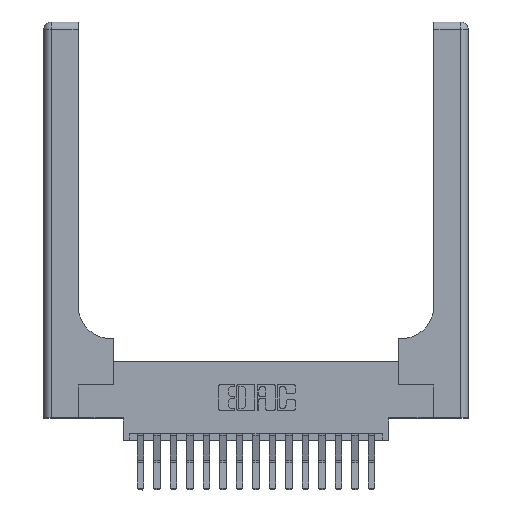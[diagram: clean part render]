
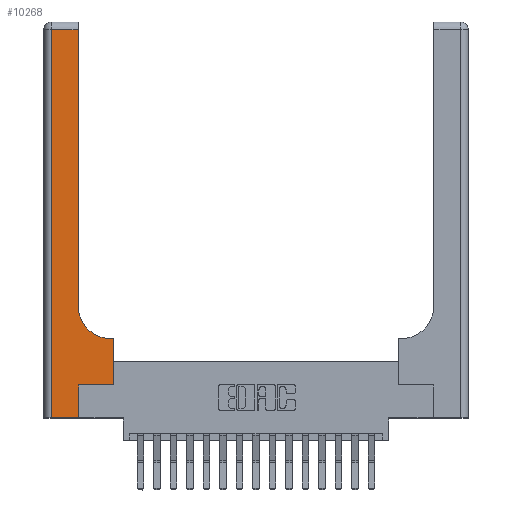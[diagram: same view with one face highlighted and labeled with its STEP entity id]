
A CAD part, top view. The second image highlights one B-rep face of the part: STEP entity #10268.
In plain terms, the highlighted planar face has unit normal (0, 0, 1).
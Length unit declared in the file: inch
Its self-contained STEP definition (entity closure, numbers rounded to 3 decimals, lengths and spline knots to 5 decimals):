
#147 = DIRECTION ( 'NONE',  ( 0., -1., 0. ) ) ;
#744 = VECTOR ( 'NONE', #9553, 39.37008 ) ;
#833 = CARTESIAN_POINT ( 'NONE',  ( 0.26, 3., 0.37 ) ) ;
#1246 = DIRECTION ( 'NONE',  ( 0., 0., -1. ) ) ;
#1381 = ORIENTED_EDGE ( 'NONE', *, *, #14808, .T. ) ;
#1442 = EDGE_CURVE ( 'NONE', #13947, #11285, #6723, .T. ) ;
#1476 = CARTESIAN_POINT ( 'NONE',  ( 0.06, 0., 0.37 ) ) ;
#1815 = PLANE ( 'NONE',  #3888 ) ;
#2178 = EDGE_CURVE ( 'NONE', #14113, #13947, #17571, .T. ) ;
#2412 = EDGE_CURVE ( 'NONE', #15582, #16375, #18259, .T. ) ;
#2527 = ORIENTED_EDGE ( 'NONE', *, *, #2178, .T. ) ;
#2862 = EDGE_LOOP ( 'NONE', ( #9346, #1381, #17458, #18027, #9876, #2527, #17839, #12191, #4688 ) ) ;
#3474 = CARTESIAN_POINT ( 'NONE',  ( 0.528, 0.6, 0.37 ) ) ;
#3888 = AXIS2_PLACEMENT_3D ( 'NONE', #7585, #4747, #14884 ) ;
#4025 = CARTESIAN_POINT ( 'NONE',  ( 0.265, 0.25, 0.37 ) ) ;
#4511 = VERTEX_POINT ( 'NONE', #5533 ) ;
#4688 = ORIENTED_EDGE ( 'NONE', *, *, #8711, .T. ) ;
#4747 = DIRECTION ( 'NONE',  ( 0., 0., -1. ) ) ;
#5014 = CIRCLE ( 'NONE', #16731, 0.25 ) ;
#5480 = DIRECTION ( 'NONE',  ( -1., 0., 0. ) ) ;
#5533 = CARTESIAN_POINT ( 'NONE',  ( 0.51, 0.6, 0.37 ) ) ;
#5555 = VECTOR ( 'NONE', #9409, 39.37008 ) ;
#6585 = VECTOR ( 'NONE', #15276, 39.37008 ) ;
#6723 = LINE ( 'NONE', #7310, #13954 ) ;
#6951 = VERTEX_POINT ( 'NONE', #13316 ) ;
#7310 = CARTESIAN_POINT ( 'NONE',  ( 0.528, 0.25, 0.37 ) ) ;
#7493 = VECTOR ( 'NONE', #10133, 39.37008 ) ;
#7585 = CARTESIAN_POINT ( 'NONE',  ( 0., 3., 0.37 ) ) ;
#7947 = CARTESIAN_POINT ( 'NONE',  ( 0., 2.94, 0.37 ) ) ;
#8485 = LINE ( 'NONE', #833, #744 ) ;
#8711 = EDGE_CURVE ( 'NONE', #4511, #6951, #5014, .T. ) ;
#8758 = DIRECTION ( 'NONE',  ( 0., 1., 0. ) ) ;
#8772 = EDGE_CURVE ( 'NONE', #16375, #16085, #11383, .T. ) ;
#9346 = ORIENTED_EDGE ( 'NONE', *, *, #14858, .T. ) ;
#9409 = DIRECTION ( 'NONE',  ( -1., 0., 0. ) ) ;
#9507 = LINE ( 'NONE', #14149, #17238 ) ;
#9553 = DIRECTION ( 'NONE',  ( 0., 1., 0. ) ) ;
#9876 = ORIENTED_EDGE ( 'NONE', *, *, #18252, .T. ) ;
#9920 = EDGE_CURVE ( 'NONE', #11285, #4511, #9507, .T. ) ;
#9958 = CARTESIAN_POINT ( 'NONE',  ( 0.51, 0.85, 0.37 ) ) ;
#10133 = DIRECTION ( 'NONE',  ( 1., 0., 0. ) ) ;
#10268 = ADVANCED_FACE ( 'NONE', ( #16074 ), #1815, .F. ) ;
#11285 = VERTEX_POINT ( 'NONE', #3474 ) ;
#11383 = LINE ( 'NONE', #18833, #7493 ) ;
#11421 = DIRECTION ( 'NONE',  ( 1., 0., 0. ) ) ;
#11519 = VERTEX_POINT ( 'NONE', #17120 ) ;
#12191 = ORIENTED_EDGE ( 'NONE', *, *, #9920, .T. ) ;
#12366 = CARTESIAN_POINT ( 'NONE',  ( 0.265, 0., 0.37 ) ) ;
#13232 = LINE ( 'NONE', #7947, #5555 ) ;
#13316 = CARTESIAN_POINT ( 'NONE',  ( 0.26, 0.85, 0.37 ) ) ;
#13947 = VERTEX_POINT ( 'NONE', #18043 ) ;
#13954 = VECTOR ( 'NONE', #8758, 39.37008 ) ;
#14024 = CARTESIAN_POINT ( 'NONE',  ( 0.265, 0.25, 0.37 ) ) ;
#14113 = VERTEX_POINT ( 'NONE', #14024 ) ;
#14149 = CARTESIAN_POINT ( 'NONE',  ( 0.26, 0.6, 0.37 ) ) ;
#14155 = DIRECTION ( 'NONE',  ( 1., 0., 0. ) ) ;
#14165 = VECTOR ( 'NONE', #14155, 39.37008 ) ;
#14808 = EDGE_CURVE ( 'NONE', #11519, #15582, #13232, .T. ) ;
#14858 = EDGE_CURVE ( 'NONE', #6951, #11519, #8485, .T. ) ;
#14884 = DIRECTION ( 'NONE',  ( -1., 0., 0. ) ) ;
#15276 = DIRECTION ( 'NONE',  ( 0., 1., 0. ) ) ;
#15388 = CARTESIAN_POINT ( 'NONE',  ( 0.265, 0., 0.37 ) ) ;
#15548 = CARTESIAN_POINT ( 'NONE',  ( 0.06, 2.94, 0.37 ) ) ;
#15582 = VERTEX_POINT ( 'NONE', #15548 ) ;
#16074 = FACE_OUTER_BOUND ( 'NONE', #2862, .T. ) ;
#16085 = VERTEX_POINT ( 'NONE', #15388 ) ;
#16375 = VERTEX_POINT ( 'NONE', #1476 ) ;
#16731 = AXIS2_PLACEMENT_3D ( 'NONE', #9958, #1246, #11421 ) ;
#17120 = CARTESIAN_POINT ( 'NONE',  ( 0.26, 2.94, 0.37 ) ) ;
#17238 = VECTOR ( 'NONE', #5480, 39.37008 ) ;
#17458 = ORIENTED_EDGE ( 'NONE', *, *, #2412, .T. ) ;
#17571 = LINE ( 'NONE', #4025, #14165 ) ;
#17574 = CARTESIAN_POINT ( 'NONE',  ( 0.06, 3., 0.37 ) ) ;
#17790 = VECTOR ( 'NONE', #147, 39.37008 ) ;
#17839 = ORIENTED_EDGE ( 'NONE', *, *, #1442, .T. ) ;
#18027 = ORIENTED_EDGE ( 'NONE', *, *, #8772, .T. ) ;
#18043 = CARTESIAN_POINT ( 'NONE',  ( 0.528, 0.25, 0.37 ) ) ;
#18162 = LINE ( 'NONE', #12366, #6585 ) ;
#18252 = EDGE_CURVE ( 'NONE', #16085, #14113, #18162, .T. ) ;
#18259 = LINE ( 'NONE', #17574, #17790 ) ;
#18833 = CARTESIAN_POINT ( 'NONE',  ( 0., 0., 0.37 ) ) ;
